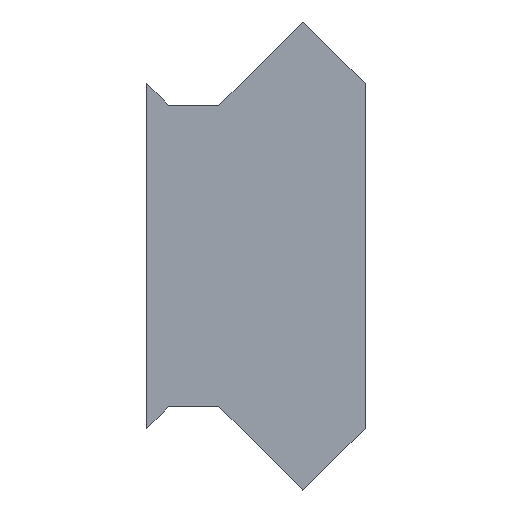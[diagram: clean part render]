
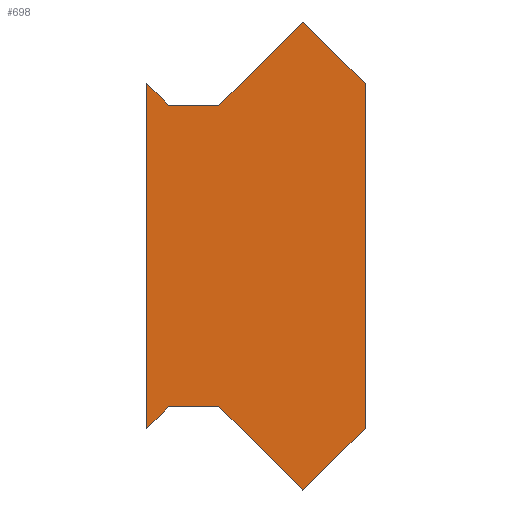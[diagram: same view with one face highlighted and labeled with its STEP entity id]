
A CAD part, left-side view. The second image highlights one B-rep face of the part: STEP entity #698.
In plain terms, the highlighted planar face has unit normal (-1, 0, 0).
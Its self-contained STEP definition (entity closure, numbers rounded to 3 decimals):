
#13 = CARTESIAN_POINT ( 'NONE',  ( 24.509, -3.133, 4.923 ) ) ;
#17 = VECTOR ( 'NONE', #1678, 1000. ) ;
#26 = DIRECTION ( 'NONE',  ( 0., 0., -1. ) ) ;
#32 = CARTESIAN_POINT ( 'NONE',  ( 24.509, -10.771, -7.563 ) ) ;
#45 = ORIENTED_EDGE ( 'NONE', *, *, #1089, .F. ) ;
#82 = LINE ( 'NONE', #146, #1423 ) ;
#131 = VERTEX_POINT ( 'NONE', #1527 ) ;
#137 = LINE ( 'NONE', #13, #555 ) ;
#146 = CARTESIAN_POINT ( 'NONE',  ( 24.509, -3.128, -4.921 ) ) ;
#152 = CARTESIAN_POINT ( 'NONE',  ( 24.509, -7.28, -11.022 ) ) ;
#193 = LINE ( 'NONE', #923, #1622 ) ;
#259 = CARTESIAN_POINT ( 'NONE',  ( 24.509, -7.28, 11.028 ) ) ;
#287 = CARTESIAN_POINT ( 'NONE',  ( 24.509, -10.22, -8.109 ) ) ;
#289 = LINE ( 'NONE', #1662, #17 ) ;
#290 = VECTOR ( 'NONE', #1338, 1000. ) ;
#295 = EDGE_CURVE ( 'NONE', #589, #1476, #289, .T. ) ;
#312 = PLANE ( 'NONE',  #833 ) ;
#318 = CARTESIAN_POINT ( 'NONE',  ( 24.509, -3.59, -0.007 ) ) ;
#336 = EDGE_CURVE ( 'NONE', #1146, #589, #1304, .T. ) ;
#349 = VECTOR ( 'NONE', #1636, 1000. ) ;
#355 = ORIENTED_EDGE ( 'NONE', *, *, #336, .F. ) ;
#387 = EDGE_CURVE ( 'NONE', #1020, #1146, #137, .T. ) ;
#407 = LINE ( 'NONE', #633, #646 ) ;
#408 = ORIENTED_EDGE ( 'NONE', *, *, #1281, .F. ) ;
#416 = VECTOR ( 'NONE', #1449, 1000. ) ;
#430 = DIRECTION ( 'NONE',  ( 0., 0.71, 0.704 ) ) ;
#433 = LINE ( 'NONE', #445, #1330 ) ;
#439 = DIRECTION ( 'NONE',  ( 0., 0., 1. ) ) ;
#445 = CARTESIAN_POINT ( 'NONE',  ( 24.509, -10.771, 7.57 ) ) ;
#447 = EDGE_CURVE ( 'NONE', #1020, #943, #193, .T. ) ;
#459 = ORIENTED_EDGE ( 'NONE', *, *, #387, .F. ) ;
#466 = VERTEX_POINT ( 'NONE', #152 ) ;
#478 = EDGE_CURVE ( 'NONE', #466, #1252, #881, .T. ) ;
#492 = DIRECTION ( 'NONE',  ( 0., -1., 0. ) ) ;
#522 = ORIENTED_EDGE ( 'NONE', *, *, #1397, .F. ) ;
#546 = ORIENTED_EDGE ( 'NONE', *, *, #447, .T. ) ;
#555 = VECTOR ( 'NONE', #650, 1000. ) ;
#558 = FACE_OUTER_BOUND ( 'NONE', #1454, .T. ) ;
#580 = CARTESIAN_POINT ( 'NONE',  ( 24.509, -10.22, 0.003 ) ) ;
#589 = VERTEX_POINT ( 'NONE', #711 ) ;
#595 = EDGE_CURVE ( 'NONE', #1287, #1476, #433, .T. ) ;
#633 = CARTESIAN_POINT ( 'NONE',  ( 24.509, -5.023, -7.109 ) ) ;
#646 = VECTOR ( 'NONE', #788, 1000. ) ;
#650 = DIRECTION ( 'NONE',  ( 0., -0.707, -0.707 ) ) ;
#698 = ADVANCED_FACE ( 'NONE', ( #558 ), #312, .F. ) ;
#711 = CARTESIAN_POINT ( 'NONE',  ( 24.509, -3.33, 7.116 ) ) ;
#788 = DIRECTION ( 'NONE',  ( 0., 1., 0. ) ) ;
#792 = VECTOR ( 'NONE', #492, 1000. ) ;
#828 = ORIENTED_EDGE ( 'NONE', *, *, #595, .T. ) ;
#833 = AXIS2_PLACEMENT_3D ( 'NONE', #318, #1632, #439 ) ;
#844 = VERTEX_POINT ( 'NONE', #1021 ) ;
#881 = LINE ( 'NONE', #32, #290 ) ;
#915 = CARTESIAN_POINT ( 'NONE',  ( 24.509, 0.06, -8.109 ) ) ;
#923 = CARTESIAN_POINT ( 'NONE',  ( 24.509, 0.06, 15.188 ) ) ;
#930 = DIRECTION ( 'NONE',  ( 0., 0.707, -0.707 ) ) ;
#943 = VERTEX_POINT ( 'NONE', #915 ) ;
#1020 = VERTEX_POINT ( 'NONE', #1313 ) ;
#1021 = CARTESIAN_POINT ( 'NONE',  ( 24.509, -0.94, -7.109 ) ) ;
#1078 = CARTESIAN_POINT ( 'NONE',  ( 24.509, -0.94, 7.116 ) ) ;
#1089 = EDGE_CURVE ( 'NONE', #466, #131, #1510, .T. ) ;
#1146 = VERTEX_POINT ( 'NONE', #1078 ) ;
#1156 = CARTESIAN_POINT ( 'NONE',  ( 24.509, -10.22, 8.116 ) ) ;
#1167 = CARTESIAN_POINT ( 'NONE',  ( 24.509, -5.023, 7.116 ) ) ;
#1226 = LINE ( 'NONE', #580, #349 ) ;
#1252 = VERTEX_POINT ( 'NONE', #287 ) ;
#1281 = EDGE_CURVE ( 'NONE', #131, #844, #407, .T. ) ;
#1287 = VERTEX_POINT ( 'NONE', #1156 ) ;
#1304 = LINE ( 'NONE', #1167, #792 ) ;
#1313 = CARTESIAN_POINT ( 'NONE',  ( 24.509, 0.06, 8.116 ) ) ;
#1330 = VECTOR ( 'NONE', #430, 1000. ) ;
#1338 = DIRECTION ( 'NONE',  ( 0., -0.71, 0.704 ) ) ;
#1353 = ORIENTED_EDGE ( 'NONE', *, *, #478, .T. ) ;
#1397 = EDGE_CURVE ( 'NONE', #844, #943, #82, .T. ) ;
#1423 = VECTOR ( 'NONE', #930, 1000. ) ;
#1449 = DIRECTION ( 'NONE',  ( 0., 0.71, 0.704 ) ) ;
#1454 = EDGE_LOOP ( 'NONE', ( #546, #522, #408, #45, #1353, #1491, #828, #1597, #355, #459 ) ) ;
#1476 = VERTEX_POINT ( 'NONE', #259 ) ;
#1491 = ORIENTED_EDGE ( 'NONE', *, *, #1675, .T. ) ;
#1510 = LINE ( 'NONE', #1584, #416 ) ;
#1527 = CARTESIAN_POINT ( 'NONE',  ( 24.509, -3.33, -7.109 ) ) ;
#1584 = CARTESIAN_POINT ( 'NONE',  ( 24.509, -3.789, -7.563 ) ) ;
#1597 = ORIENTED_EDGE ( 'NONE', *, *, #295, .F. ) ;
#1622 = VECTOR ( 'NONE', #26, 1000. ) ;
#1632 = DIRECTION ( 'NONE',  ( 1., 0., 0. ) ) ;
#1636 = DIRECTION ( 'NONE',  ( 0., 0., 1. ) ) ;
#1662 = CARTESIAN_POINT ( 'NONE',  ( 24.509, -3.789, 7.57 ) ) ;
#1675 = EDGE_CURVE ( 'NONE', #1252, #1287, #1226, .T. ) ;
#1678 = DIRECTION ( 'NONE',  ( 0., -0.71, 0.704 ) ) ;
